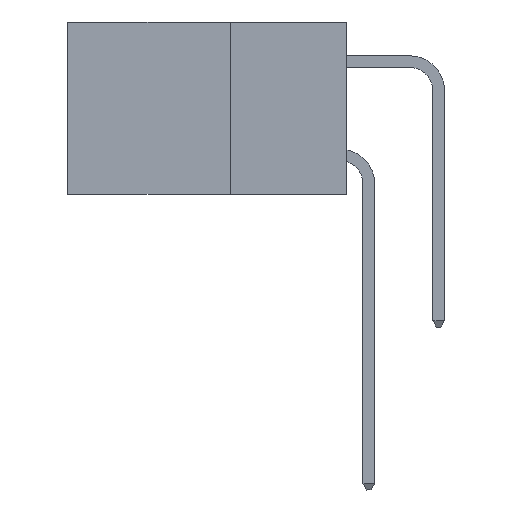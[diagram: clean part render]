
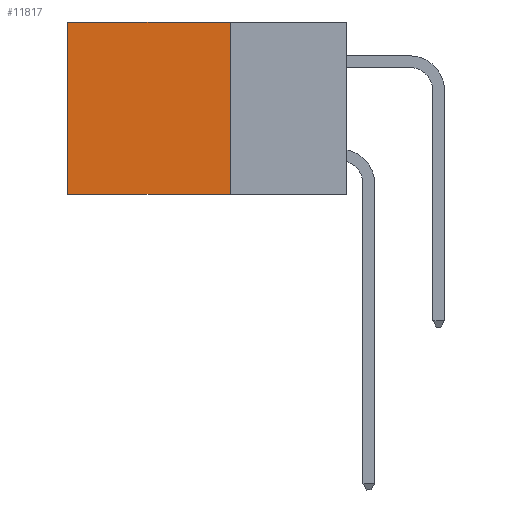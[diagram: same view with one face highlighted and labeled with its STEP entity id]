
A CAD part, left-side view. The second image highlights one B-rep face of the part: STEP entity #11817.
In plain terms, the highlighted planar face has unit normal (-1, 0, 0).
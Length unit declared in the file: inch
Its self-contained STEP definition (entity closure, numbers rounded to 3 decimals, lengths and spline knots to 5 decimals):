
#865 = FACE_OUTER_BOUND ( 'NONE', #11531, .T. ) ;
#887 = CARTESIAN_POINT ( 'NONE',  ( 0.2875, 0.6, 0. ) ) ;
#1740 = ORIENTED_EDGE ( 'NONE', *, *, #7961, .T. ) ;
#2173 = VERTEX_POINT ( 'NONE', #11889 ) ;
#2217 = VECTOR ( 'NONE', #5617, 39.37008 ) ;
#2925 = EDGE_CURVE ( 'NONE', #2173, #4551, #8231, .T. ) ;
#2939 = ORIENTED_EDGE ( 'NONE', *, *, #10514, .F. ) ;
#2970 = EDGE_CURVE ( 'NONE', #9277, #3455, #7610, .T. ) ;
#3033 = CARTESIAN_POINT ( 'NONE',  ( 0.2875, 0.6, 0. ) ) ;
#3077 = ORIENTED_EDGE ( 'NONE', *, *, #2970, .T. ) ;
#3455 = VERTEX_POINT ( 'NONE', #3033 ) ;
#4327 = VECTOR ( 'NONE', #7130, 39.37008 ) ;
#4551 = VERTEX_POINT ( 'NONE', #8267 ) ;
#4989 = VECTOR ( 'NONE', #10798, 39.37008 ) ;
#5617 = DIRECTION ( 'NONE',  ( 0., 1., 0. ) ) ;
#5630 = LINE ( 'NONE', #11750, #4989 ) ;
#5896 = DIRECTION ( 'NONE',  ( 1., 0., 0. ) ) ;
#5980 = CARTESIAN_POINT ( 'NONE',  ( 0.2875, 0.25, 0. ) ) ;
#6544 = CARTESIAN_POINT ( 'NONE',  ( 0.2875, 0.25, 0. ) ) ;
#6840 = PLANE ( 'NONE',  #9771 ) ;
#7130 = DIRECTION ( 'NONE',  ( 0., 0., -1. ) ) ;
#7610 = LINE ( 'NONE', #5980, #2217 ) ;
#7961 = EDGE_CURVE ( 'NONE', #3455, #4551, #11720, .T. ) ;
#8231 = LINE ( 'NONE', #8414, #8872 ) ;
#8267 = CARTESIAN_POINT ( 'NONE',  ( 0.2875, 0.6, -0.37 ) ) ;
#8414 = CARTESIAN_POINT ( 'NONE',  ( 0.2875, 0.25, -0.37 ) ) ;
#8698 = DIRECTION ( 'NONE',  ( 0., 1., 0. ) ) ;
#8872 = VECTOR ( 'NONE', #8698, 39.37008 ) ;
#8879 = CARTESIAN_POINT ( 'NONE',  ( 0.2875, 0.25, 0. ) ) ;
#9277 = VERTEX_POINT ( 'NONE', #6544 ) ;
#9771 = AXIS2_PLACEMENT_3D ( 'NONE', #8879, #5896, #12852 ) ;
#10514 = EDGE_CURVE ( 'NONE', #9277, #2173, #5630, .T. ) ;
#10798 = DIRECTION ( 'NONE',  ( 0., 0., -1. ) ) ;
#11531 = EDGE_LOOP ( 'NONE', ( #1740, #13081, #2939, #3077 ) ) ;
#11720 = LINE ( 'NONE', #887, #4327 ) ;
#11750 = CARTESIAN_POINT ( 'NONE',  ( 0.2875, 0.25, 0. ) ) ;
#11817 = ADVANCED_FACE ( 'NONE', ( #865 ), #6840, .F. ) ;
#11889 = CARTESIAN_POINT ( 'NONE',  ( 0.2875, 0.25, -0.37 ) ) ;
#12852 = DIRECTION ( 'NONE',  ( 0., 0., -1. ) ) ;
#13081 = ORIENTED_EDGE ( 'NONE', *, *, #2925, .F. ) ;
